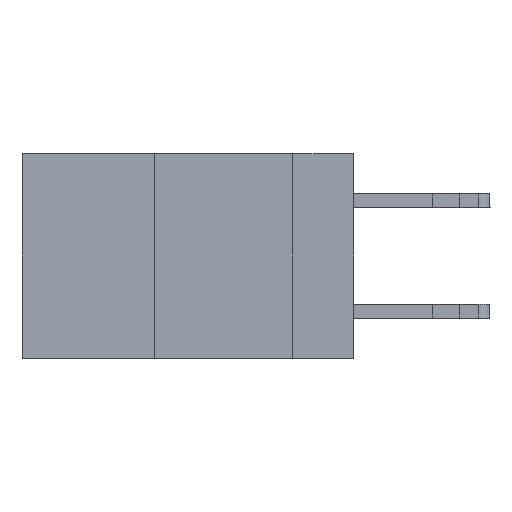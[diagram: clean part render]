
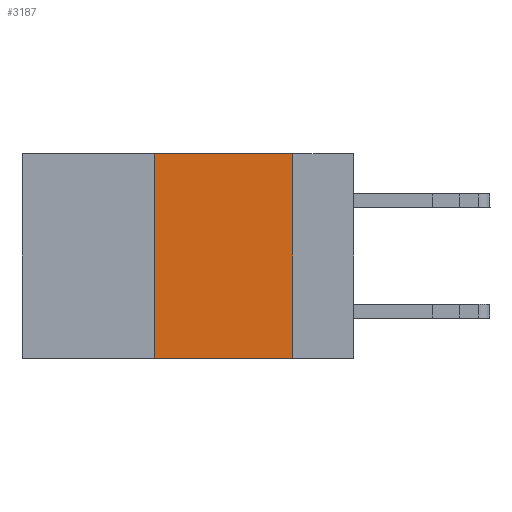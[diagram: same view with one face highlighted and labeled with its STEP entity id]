
A CAD part, left-side view. The second image highlights one B-rep face of the part: STEP entity #3187.
In plain terms, the highlighted planar face has unit normal (-1, 0, 0).
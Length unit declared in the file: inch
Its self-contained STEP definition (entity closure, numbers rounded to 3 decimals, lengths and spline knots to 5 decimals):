
#193 = VECTOR ( 'NONE', #17410, 39.37008 ) ;
#430 = VECTOR ( 'NONE', #18699, 39.37008 ) ;
#564 = ORIENTED_EDGE ( 'NONE', *, *, #4753, .F. ) ;
#1621 = DIRECTION ( 'NONE',  ( 1., 0., 0. ) ) ;
#2902 = CARTESIAN_POINT ( 'NONE',  ( 0., 0.11, -0.37 ) ) ;
#3187 = ADVANCED_FACE ( 'NONE', ( #12320 ), #13783, .F. ) ;
#3497 = EDGE_CURVE ( 'NONE', #7311, #18287, #18773, .T. ) ;
#4753 = EDGE_CURVE ( 'NONE', #18287, #18256, #18112, .T. ) ;
#6878 = CARTESIAN_POINT ( 'NONE',  ( 0., 0.36, 0. ) ) ;
#6975 = LINE ( 'NONE', #6878, #430 ) ;
#7201 = VECTOR ( 'NONE', #17166, 39.37008 ) ;
#7311 = VERTEX_POINT ( 'NONE', #15502 ) ;
#7830 = CARTESIAN_POINT ( 'NONE',  ( 0., 0.6, 0. ) ) ;
#7989 = ORIENTED_EDGE ( 'NONE', *, *, #8769, .T. ) ;
#8371 = LINE ( 'NONE', #16875, #7201 ) ;
#8570 = EDGE_LOOP ( 'NONE', ( #564, #14796, #18337, #7989 ) ) ;
#8769 = EDGE_CURVE ( 'NONE', #17721, #18256, #8371, .T. ) ;
#9242 = CARTESIAN_POINT ( 'NONE',  ( 0., 0.11, 0. ) ) ;
#9538 = VECTOR ( 'NONE', #16859, 39.37008 ) ;
#12229 = DIRECTION ( 'NONE',  ( 0., 0., -1. ) ) ;
#12320 = FACE_OUTER_BOUND ( 'NONE', #8570, .T. ) ;
#13783 = PLANE ( 'NONE',  #15759 ) ;
#14695 = CARTESIAN_POINT ( 'NONE',  ( 0., 0.11, 0. ) ) ;
#14740 = CARTESIAN_POINT ( 'NONE',  ( 0., 0.6, 0. ) ) ;
#14796 = ORIENTED_EDGE ( 'NONE', *, *, #3497, .F. ) ;
#15502 = CARTESIAN_POINT ( 'NONE',  ( 0., 0.36, 0. ) ) ;
#15759 = AXIS2_PLACEMENT_3D ( 'NONE', #7830, #1621, #12229 ) ;
#16859 = DIRECTION ( 'NONE',  ( 0., 0., -1. ) ) ;
#16875 = CARTESIAN_POINT ( 'NONE',  ( 0., 0.6, -0.37 ) ) ;
#17166 = DIRECTION ( 'NONE',  ( 0., -1., 0. ) ) ;
#17410 = DIRECTION ( 'NONE',  ( 0., -1., 0. ) ) ;
#17473 = CARTESIAN_POINT ( 'NONE',  ( 0., 0.36, -0.37 ) ) ;
#17721 = VERTEX_POINT ( 'NONE', #17473 ) ;
#18112 = LINE ( 'NONE', #9242, #9538 ) ;
#18256 = VERTEX_POINT ( 'NONE', #2902 ) ;
#18287 = VERTEX_POINT ( 'NONE', #14695 ) ;
#18337 = ORIENTED_EDGE ( 'NONE', *, *, #18566, .F. ) ;
#18566 = EDGE_CURVE ( 'NONE', #17721, #7311, #6975, .T. ) ;
#18699 = DIRECTION ( 'NONE',  ( 0., 0., 1. ) ) ;
#18773 = LINE ( 'NONE', #14740, #193 ) ;
